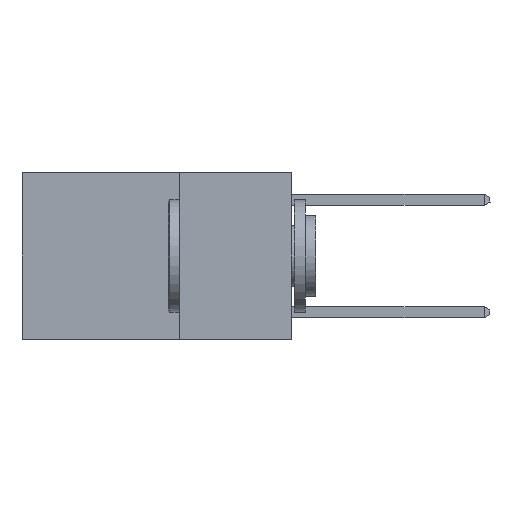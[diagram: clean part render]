
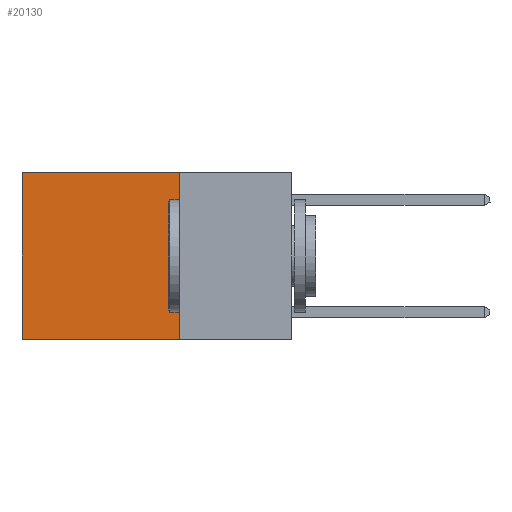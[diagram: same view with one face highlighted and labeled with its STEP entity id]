
A CAD part, left-side view. The second image highlights one B-rep face of the part: STEP entity #20130.
In plain terms, the highlighted planar face has unit normal (-1, 0, 0).
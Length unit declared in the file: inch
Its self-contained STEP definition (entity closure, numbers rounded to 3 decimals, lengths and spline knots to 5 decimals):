
#64 = DIRECTION ( 'NONE',  ( 0., 0., -1. ) ) ;
#147 = VERTEX_POINT ( 'NONE', #10527 ) ;
#171 = LINE ( 'NONE', #945, #23014 ) ;
#443 = VECTOR ( 'NONE', #18036, 39.37008 ) ;
#470 = ORIENTED_EDGE ( 'NONE', *, *, #2254, .T. ) ;
#945 = CARTESIAN_POINT ( 'NONE',  ( 0.2625, 0.25, 0. ) ) ;
#1488 = EDGE_CURVE ( 'NONE', #8915, #14290, #23272, .T. ) ;
#2210 = LINE ( 'NONE', #3561, #6506 ) ;
#2254 = EDGE_CURVE ( 'NONE', #9335, #147, #14263, .T. ) ;
#2442 = CARTESIAN_POINT ( 'NONE',  ( 0.2625, 0.25, 0. ) ) ;
#3561 = CARTESIAN_POINT ( 'NONE',  ( 0.2625, 0.6, 0. ) ) ;
#4813 = FACE_OUTER_BOUND ( 'NONE', #17652, .T. ) ;
#5203 = CARTESIAN_POINT ( 'NONE',  ( 0.2625, 0.25, -0.37 ) ) ;
#5682 = CARTESIAN_POINT ( 'NONE',  ( 0.2625, 0.25, -0.37 ) ) ;
#6209 = VECTOR ( 'NONE', #7983, 39.37008 ) ;
#6506 = VECTOR ( 'NONE', #64, 39.37008 ) ;
#7983 = DIRECTION ( 'NONE',  ( 0., 1., 0. ) ) ;
#8915 = VERTEX_POINT ( 'NONE', #5682 ) ;
#9335 = VERTEX_POINT ( 'NONE', #22305 ) ;
#10399 = ORIENTED_EDGE ( 'NONE', *, *, #16461, .T. ) ;
#10527 = CARTESIAN_POINT ( 'NONE',  ( 0.2625, 0.6, 0. ) ) ;
#11123 = ORIENTED_EDGE ( 'NONE', *, *, #1488, .F. ) ;
#12230 = DIRECTION ( 'NONE',  ( 0., 0., -1. ) ) ;
#13332 = ORIENTED_EDGE ( 'NONE', *, *, #20637, .F. ) ;
#13817 = DIRECTION ( 'NONE',  ( 0., 0., -1. ) ) ;
#14263 = LINE ( 'NONE', #2442, #6209 ) ;
#14290 = VERTEX_POINT ( 'NONE', #19794 ) ;
#15589 = AXIS2_PLACEMENT_3D ( 'NONE', #19374, #21503, #12230 ) ;
#16461 = EDGE_CURVE ( 'NONE', #147, #14290, #2210, .T. ) ;
#17652 = EDGE_LOOP ( 'NONE', ( #10399, #11123, #13332, #470 ) ) ;
#18036 = DIRECTION ( 'NONE',  ( 0., 1., 0. ) ) ;
#19374 = CARTESIAN_POINT ( 'NONE',  ( 0.2625, 0.25, 0. ) ) ;
#19616 = PLANE ( 'NONE',  #15589 ) ;
#19794 = CARTESIAN_POINT ( 'NONE',  ( 0.2625, 0.6, -0.37 ) ) ;
#20130 = ADVANCED_FACE ( 'NONE', ( #4813 ), #19616, .F. ) ;
#20637 = EDGE_CURVE ( 'NONE', #9335, #8915, #171, .T. ) ;
#21503 = DIRECTION ( 'NONE',  ( 1., 0., 0. ) ) ;
#22305 = CARTESIAN_POINT ( 'NONE',  ( 0.2625, 0.25, 0. ) ) ;
#23014 = VECTOR ( 'NONE', #13817, 39.37008 ) ;
#23272 = LINE ( 'NONE', #5203, #443 ) ;
